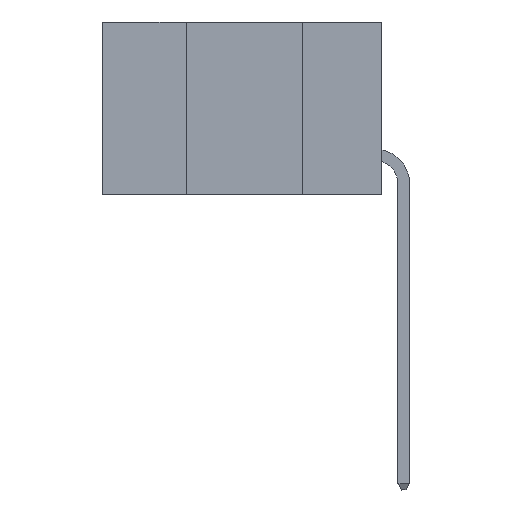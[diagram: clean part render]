
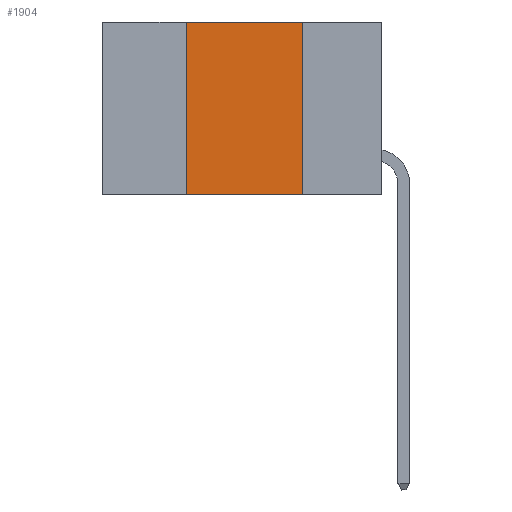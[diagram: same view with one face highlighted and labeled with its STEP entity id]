
A CAD part, left-side view. The second image highlights one B-rep face of the part: STEP entity #1904.
In plain terms, the highlighted planar face has unit normal (-1, 0, 0).
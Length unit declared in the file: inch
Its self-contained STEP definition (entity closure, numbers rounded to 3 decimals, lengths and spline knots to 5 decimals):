
#758 = EDGE_CURVE ( 'NONE', #6534, #10608, #23911, .T. ) ;
#1605 = EDGE_CURVE ( 'NONE', #18096, #10608, #6597, .T. ) ;
#1904 = ADVANCED_FACE ( 'NONE', ( #14477 ), #15979, .F. ) ;
#2008 = CARTESIAN_POINT ( 'NONE',  ( 0., 0.6, 0. ) ) ;
#4988 = VECTOR ( 'NONE', #14875, 39.37008 ) ;
#5157 = DIRECTION ( 'NONE',  ( 0., 0., -1. ) ) ;
#6534 = VERTEX_POINT ( 'NONE', #11311 ) ;
#6597 = LINE ( 'NONE', #13826, #26279 ) ;
#6749 = CARTESIAN_POINT ( 'NONE',  ( 0., 0.17, -0.37 ) ) ;
#7113 = CARTESIAN_POINT ( 'NONE',  ( 0., 0.6, 0. ) ) ;
#7198 = DIRECTION ( 'NONE',  ( 0., 0., -1. ) ) ;
#9763 = ORIENTED_EDGE ( 'NONE', *, *, #20690, .F. ) ;
#10438 = CARTESIAN_POINT ( 'NONE',  ( 0., 0.42, 0. ) ) ;
#10456 = ORIENTED_EDGE ( 'NONE', *, *, #1605, .F. ) ;
#10608 = VERTEX_POINT ( 'NONE', #6749 ) ;
#10617 = DIRECTION ( 'NONE',  ( 0., -1., 0. ) ) ;
#10797 = DIRECTION ( 'NONE',  ( 0., -1., 0. ) ) ;
#11311 = CARTESIAN_POINT ( 'NONE',  ( 0., 0.42, -0.37 ) ) ;
#13826 = CARTESIAN_POINT ( 'NONE',  ( 0., 0.17, 0. ) ) ;
#14477 = FACE_OUTER_BOUND ( 'NONE', #21968, .T. ) ;
#14875 = DIRECTION ( 'NONE',  ( 0., 0., 1. ) ) ;
#15381 = AXIS2_PLACEMENT_3D ( 'NONE', #7113, #20686, #5157 ) ;
#15979 = PLANE ( 'NONE',  #15381 ) ;
#18096 = VERTEX_POINT ( 'NONE', #28001 ) ;
#18407 = CARTESIAN_POINT ( 'NONE',  ( 0., 0.42, 0. ) ) ;
#18619 = VECTOR ( 'NONE', #10617, 39.37008 ) ;
#18699 = VECTOR ( 'NONE', #10797, 39.37008 ) ;
#19140 = LINE ( 'NONE', #10438, #4988 ) ;
#19846 = ORIENTED_EDGE ( 'NONE', *, *, #758, .T. ) ;
#20686 = DIRECTION ( 'NONE',  ( 1., 0., 0. ) ) ;
#20690 = EDGE_CURVE ( 'NONE', #23671, #18096, #25202, .T. ) ;
#21968 = EDGE_LOOP ( 'NONE', ( #10456, #9763, #28347, #19846 ) ) ;
#23671 = VERTEX_POINT ( 'NONE', #18407 ) ;
#23911 = LINE ( 'NONE', #28169, #18699 ) ;
#25202 = LINE ( 'NONE', #2008, #18619 ) ;
#26279 = VECTOR ( 'NONE', #7198, 39.37008 ) ;
#27122 = EDGE_CURVE ( 'NONE', #6534, #23671, #19140, .T. ) ;
#28001 = CARTESIAN_POINT ( 'NONE',  ( 0., 0.17, 0. ) ) ;
#28169 = CARTESIAN_POINT ( 'NONE',  ( 0., 0.6, -0.37 ) ) ;
#28347 = ORIENTED_EDGE ( 'NONE', *, *, #27122, .F. ) ;
